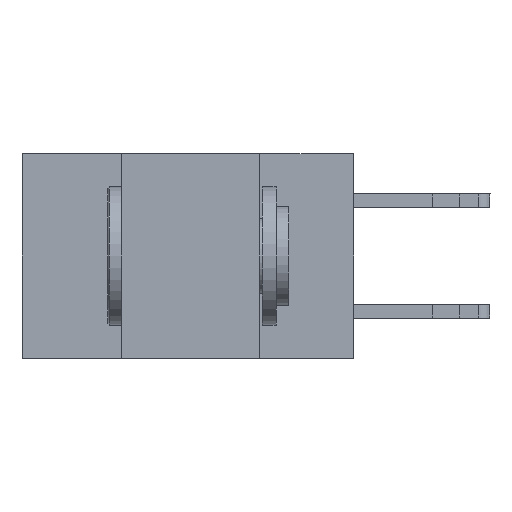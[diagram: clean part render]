
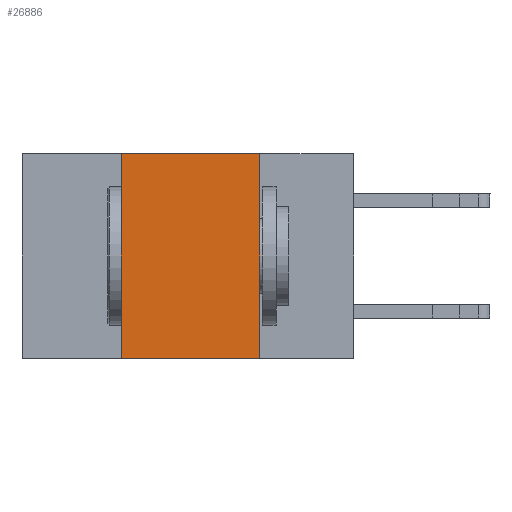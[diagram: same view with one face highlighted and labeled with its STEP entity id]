
A CAD part, left-side view. The second image highlights one B-rep face of the part: STEP entity #26886.
In plain terms, the highlighted planar face has unit normal (-1, 0, 0).
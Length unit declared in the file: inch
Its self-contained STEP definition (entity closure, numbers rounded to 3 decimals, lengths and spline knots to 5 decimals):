
#2866 = LINE ( 'NONE', #3791, #7546 ) ;
#2872 = AXIS2_PLACEMENT_3D ( 'NONE', #12601, #31693, #20939 ) ;
#3222 = VERTEX_POINT ( 'NONE', #22040 ) ;
#3528 = VECTOR ( 'NONE', #25577, 39.37008 ) ;
#3636 = VERTEX_POINT ( 'NONE', #19798 ) ;
#3791 = CARTESIAN_POINT ( 'NONE',  ( 0., 0.6, 0. ) ) ;
#4614 = CARTESIAN_POINT ( 'NONE',  ( 0., 0.42, 0. ) ) ;
#5162 = CARTESIAN_POINT ( 'NONE',  ( 0., 0.17, 0. ) ) ;
#7546 = VECTOR ( 'NONE', #17156, 39.37008 ) ;
#8855 = VECTOR ( 'NONE', #20633, 39.37008 ) ;
#9050 = ORIENTED_EDGE ( 'NONE', *, *, #15038, .F. ) ;
#9455 = VERTEX_POINT ( 'NONE', #24684 ) ;
#9741 = CARTESIAN_POINT ( 'NONE',  ( 0., 0.42, -0.37 ) ) ;
#10924 = VERTEX_POINT ( 'NONE', #9741 ) ;
#11357 = EDGE_CURVE ( 'NONE', #3636, #3222, #21688, .T. ) ;
#12601 = CARTESIAN_POINT ( 'NONE',  ( 0., 0.6, 0. ) ) ;
#13519 = LINE ( 'NONE', #15235, #8855 ) ;
#13682 = EDGE_LOOP ( 'NONE', ( #16724, #9050, #19950, #22516 ) ) ;
#15038 = EDGE_CURVE ( 'NONE', #9455, #3636, #2866, .T. ) ;
#15235 = CARTESIAN_POINT ( 'NONE',  ( 0., 0.6, -0.37 ) ) ;
#16724 = ORIENTED_EDGE ( 'NONE', *, *, #11357, .F. ) ;
#17156 = DIRECTION ( 'NONE',  ( 0., -1., 0. ) ) ;
#17720 = VECTOR ( 'NONE', #24083, 39.37008 ) ;
#17768 = PLANE ( 'NONE',  #2872 ) ;
#19798 = CARTESIAN_POINT ( 'NONE',  ( 0., 0.17, 0. ) ) ;
#19950 = ORIENTED_EDGE ( 'NONE', *, *, #21162, .F. ) ;
#20633 = DIRECTION ( 'NONE',  ( 0., -1., 0. ) ) ;
#20939 = DIRECTION ( 'NONE',  ( 0., 0., -1. ) ) ;
#21162 = EDGE_CURVE ( 'NONE', #10924, #9455, #26627, .T. ) ;
#21203 = EDGE_CURVE ( 'NONE', #10924, #3222, #13519, .T. ) ;
#21688 = LINE ( 'NONE', #5162, #3528 ) ;
#22040 = CARTESIAN_POINT ( 'NONE',  ( 0., 0.17, -0.37 ) ) ;
#22516 = ORIENTED_EDGE ( 'NONE', *, *, #21203, .T. ) ;
#24083 = DIRECTION ( 'NONE',  ( 0., 0., 1. ) ) ;
#24684 = CARTESIAN_POINT ( 'NONE',  ( 0., 0.42, 0. ) ) ;
#25577 = DIRECTION ( 'NONE',  ( 0., 0., -1. ) ) ;
#26627 = LINE ( 'NONE', #4614, #17720 ) ;
#26886 = ADVANCED_FACE ( 'NONE', ( #34471 ), #17768, .F. ) ;
#31693 = DIRECTION ( 'NONE',  ( 1., 0., 0. ) ) ;
#34471 = FACE_OUTER_BOUND ( 'NONE', #13682, .T. ) ;
